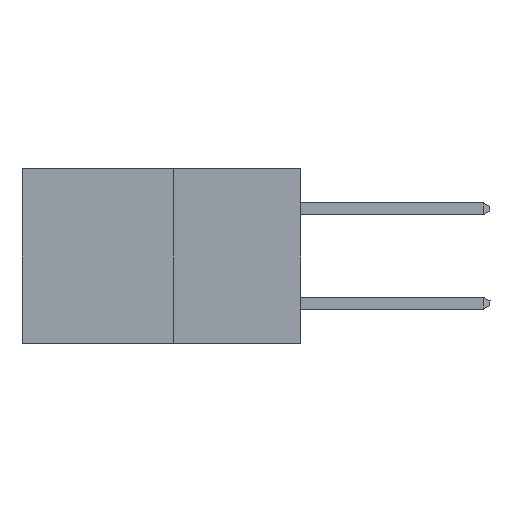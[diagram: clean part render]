
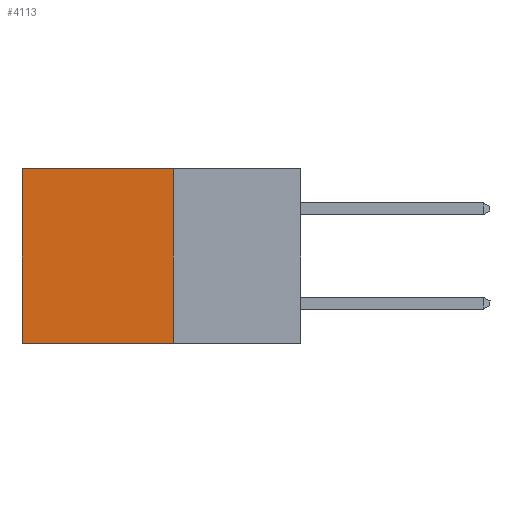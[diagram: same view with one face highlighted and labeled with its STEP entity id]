
A CAD part, left-side view. The second image highlights one B-rep face of the part: STEP entity #4113.
In plain terms, the highlighted planar face has unit normal (-1, 0, 0).
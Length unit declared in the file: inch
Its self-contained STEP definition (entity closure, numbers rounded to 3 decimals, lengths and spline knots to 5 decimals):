
#86 = VERTEX_POINT ( 'NONE', #4262 ) ;
#374 = VERTEX_POINT ( 'NONE', #8020 ) ;
#608 = LINE ( 'NONE', #5208, #4956 ) ;
#913 = VERTEX_POINT ( 'NONE', #4491 ) ;
#936 = EDGE_CURVE ( 'NONE', #913, #374, #608, .T. ) ;
#1260 = PLANE ( 'NONE',  #1470 ) ;
#1353 = CARTESIAN_POINT ( 'NONE',  ( 0.277, 0.27, -0.37 ) ) ;
#1470 = AXIS2_PLACEMENT_3D ( 'NONE', #1353, #6712, #2237 ) ;
#1494 = FACE_OUTER_BOUND ( 'NONE', #1783, .T. ) ;
#1737 = EDGE_CURVE ( 'NONE', #5900, #86, #7870, .T. ) ;
#1783 = EDGE_LOOP ( 'NONE', ( #3516, #2472, #7699, #5328 ) ) ;
#1835 = EDGE_CURVE ( 'NONE', #86, #374, #6969, .T. ) ;
#1912 = VECTOR ( 'NONE', #5526, 39.37008 ) ;
#2237 = DIRECTION ( 'NONE',  ( 0., 0., -1. ) ) ;
#2472 = ORIENTED_EDGE ( 'NONE', *, *, #936, .F. ) ;
#2990 = EDGE_CURVE ( 'NONE', #5900, #913, #6303, .T. ) ;
#3516 = ORIENTED_EDGE ( 'NONE', *, *, #1835, .T. ) ;
#4113 = ADVANCED_FACE ( 'NONE', ( #1494 ), #1260, .F. ) ;
#4175 = DIRECTION ( 'NONE',  ( 0., 0., -1. ) ) ;
#4262 = CARTESIAN_POINT ( 'NONE',  ( 0.277, 0.59, 0. ) ) ;
#4491 = CARTESIAN_POINT ( 'NONE',  ( 0.277, 0.27, -0.37 ) ) ;
#4956 = VECTOR ( 'NONE', #6556, 39.37008 ) ;
#4995 = VECTOR ( 'NONE', #4175, 39.37008 ) ;
#5208 = CARTESIAN_POINT ( 'NONE',  ( 0.277, 0.27, -0.37 ) ) ;
#5267 = CARTESIAN_POINT ( 'NONE',  ( 0.277, 0.59, -0.37 ) ) ;
#5328 = ORIENTED_EDGE ( 'NONE', *, *, #1737, .T. ) ;
#5465 = CARTESIAN_POINT ( 'NONE',  ( 0.277, 0.27, 0. ) ) ;
#5526 = DIRECTION ( 'NONE',  ( 0., 1., 0. ) ) ;
#5900 = VERTEX_POINT ( 'NONE', #7060 ) ;
#6113 = CARTESIAN_POINT ( 'NONE',  ( 0.277, 0.27, -0.37 ) ) ;
#6303 = LINE ( 'NONE', #6113, #7798 ) ;
#6556 = DIRECTION ( 'NONE',  ( 0., 1., 0. ) ) ;
#6712 = DIRECTION ( 'NONE',  ( 1., 0., 0. ) ) ;
#6969 = LINE ( 'NONE', #5267, #4995 ) ;
#7060 = CARTESIAN_POINT ( 'NONE',  ( 0.277, 0.27, 0. ) ) ;
#7699 = ORIENTED_EDGE ( 'NONE', *, *, #2990, .F. ) ;
#7798 = VECTOR ( 'NONE', #9167, 39.37008 ) ;
#7870 = LINE ( 'NONE', #5465, #1912 ) ;
#8020 = CARTESIAN_POINT ( 'NONE',  ( 0.277, 0.59, -0.37 ) ) ;
#9167 = DIRECTION ( 'NONE',  ( 0., 0., -1. ) ) ;
